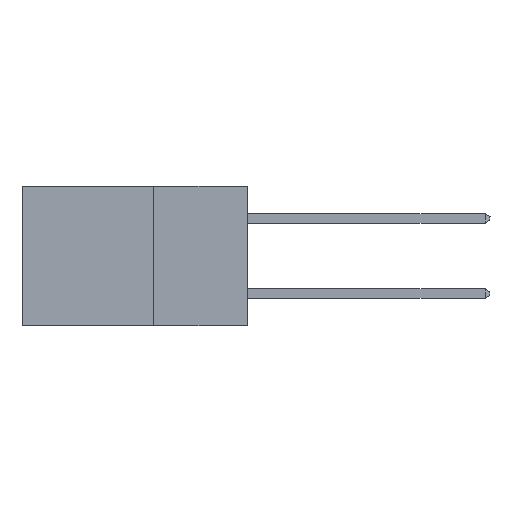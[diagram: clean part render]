
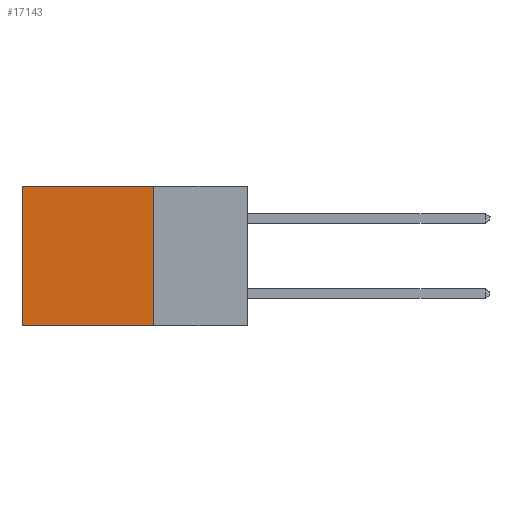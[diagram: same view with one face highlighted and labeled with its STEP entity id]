
A CAD part, left-side view. The second image highlights one B-rep face of the part: STEP entity #17143.
In plain terms, the highlighted planar face has unit normal (-1, 0, 0).
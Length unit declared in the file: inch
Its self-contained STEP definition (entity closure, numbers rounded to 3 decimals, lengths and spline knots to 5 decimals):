
#383 = DIRECTION ( 'NONE',  ( 0., 1., 0. ) ) ;
#548 = DIRECTION ( 'NONE',  ( 0., 1., 0. ) ) ;
#1680 = EDGE_CURVE ( 'NONE', #12721, #7023, #9432, .T. ) ;
#3194 = PLANE ( 'NONE',  #13418 ) ;
#3256 = CARTESIAN_POINT ( 'NONE',  ( 0.298, 0.6, 0. ) ) ;
#5279 = VERTEX_POINT ( 'NONE', #23298 ) ;
#5434 = DIRECTION ( 'NONE',  ( 0., 0., -1. ) ) ;
#5988 = CARTESIAN_POINT ( 'NONE',  ( 0.298, 0.25, -0.37 ) ) ;
#6045 = VERTEX_POINT ( 'NONE', #5988 ) ;
#7023 = VERTEX_POINT ( 'NONE', #22674 ) ;
#7319 = EDGE_LOOP ( 'NONE', ( #8615, #26384, #10927, #11495 ) ) ;
#8458 = EDGE_CURVE ( 'NONE', #5279, #12721, #26500, .T. ) ;
#8615 = ORIENTED_EDGE ( 'NONE', *, *, #1680, .T. ) ;
#9432 = LINE ( 'NONE', #25219, #18350 ) ;
#10026 = VECTOR ( 'NONE', #383, 39.37008 ) ;
#10927 = ORIENTED_EDGE ( 'NONE', *, *, #20488, .F. ) ;
#11440 = LINE ( 'NONE', #21919, #27320 ) ;
#11495 = ORIENTED_EDGE ( 'NONE', *, *, #8458, .T. ) ;
#11921 = CARTESIAN_POINT ( 'NONE',  ( 0.298, 0.25, 0. ) ) ;
#12721 = VERTEX_POINT ( 'NONE', #3256 ) ;
#13418 = AXIS2_PLACEMENT_3D ( 'NONE', #11921, #18094, #5434 ) ;
#15771 = DIRECTION ( 'NONE',  ( 0., 0., -1. ) ) ;
#17143 = ADVANCED_FACE ( 'NONE', ( #19418 ), #3194, .F. ) ;
#18094 = DIRECTION ( 'NONE',  ( 1., 0., 0. ) ) ;
#18350 = VECTOR ( 'NONE', #27407, 39.37008 ) ;
#19418 = FACE_OUTER_BOUND ( 'NONE', #7319, .T. ) ;
#20488 = EDGE_CURVE ( 'NONE', #5279, #6045, #11440, .T. ) ;
#21178 = VECTOR ( 'NONE', #548, 39.37008 ) ;
#21919 = CARTESIAN_POINT ( 'NONE',  ( 0.298, 0.25, 0. ) ) ;
#22674 = CARTESIAN_POINT ( 'NONE',  ( 0.298, 0.6, -0.37 ) ) ;
#23298 = CARTESIAN_POINT ( 'NONE',  ( 0.298, 0.25, 0. ) ) ;
#23751 = CARTESIAN_POINT ( 'NONE',  ( 0.298, 0.25, 0. ) ) ;
#23772 = CARTESIAN_POINT ( 'NONE',  ( 0.298, 0.25, -0.37 ) ) ;
#24287 = LINE ( 'NONE', #23772, #10026 ) ;
#25219 = CARTESIAN_POINT ( 'NONE',  ( 0.298, 0.6, 0. ) ) ;
#26384 = ORIENTED_EDGE ( 'NONE', *, *, #26435, .F. ) ;
#26435 = EDGE_CURVE ( 'NONE', #6045, #7023, #24287, .T. ) ;
#26500 = LINE ( 'NONE', #23751, #21178 ) ;
#27320 = VECTOR ( 'NONE', #15771, 39.37008 ) ;
#27407 = DIRECTION ( 'NONE',  ( 0., 0., -1. ) ) ;
